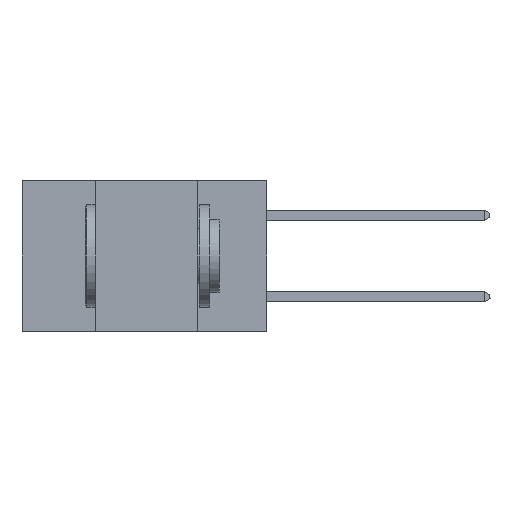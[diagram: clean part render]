
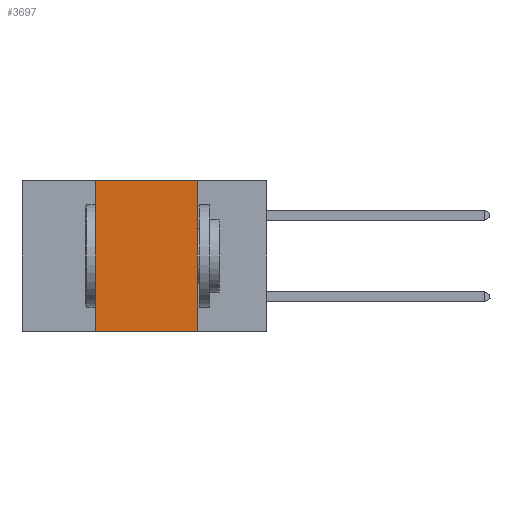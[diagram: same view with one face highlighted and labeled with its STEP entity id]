
A CAD part, left-side view. The second image highlights one B-rep face of the part: STEP entity #3697.
In plain terms, the highlighted planar face has unit normal (-1, 0, 0).
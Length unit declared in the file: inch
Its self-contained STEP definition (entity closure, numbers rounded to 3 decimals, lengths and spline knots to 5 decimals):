
#259 = DIRECTION ( 'NONE',  ( 1., 0., 0. ) ) ;
#348 = PLANE ( 'NONE',  #26039 ) ;
#994 = DIRECTION ( 'NONE',  ( 0., -1., 0. ) ) ;
#1923 = VERTEX_POINT ( 'NONE', #11440 ) ;
#2214 = ORIENTED_EDGE ( 'NONE', *, *, #6270, .T. ) ;
#3105 = DIRECTION ( 'NONE',  ( 0., 0., 1. ) ) ;
#3697 = ADVANCED_FACE ( 'NONE', ( #11895 ), #348, .F. ) ;
#4535 = DIRECTION ( 'NONE',  ( 0., 0., -1. ) ) ;
#4853 = VECTOR ( 'NONE', #19238, 39.37008 ) ;
#4961 = VECTOR ( 'NONE', #12912, 39.37008 ) ;
#5135 = CARTESIAN_POINT ( 'NONE',  ( 0., 0.42, 0. ) ) ;
#5522 = VERTEX_POINT ( 'NONE', #5718 ) ;
#5718 = CARTESIAN_POINT ( 'NONE',  ( 0., 0.17, 0. ) ) ;
#6270 = EDGE_CURVE ( 'NONE', #17530, #27174, #6605, .T. ) ;
#6420 = VECTOR ( 'NONE', #3105, 39.37008 ) ;
#6551 = EDGE_CURVE ( 'NONE', #5522, #27174, #23052, .T. ) ;
#6605 = LINE ( 'NONE', #9793, #17155 ) ;
#6617 = CARTESIAN_POINT ( 'NONE',  ( 0., 0.17, -0.37 ) ) ;
#8066 = CARTESIAN_POINT ( 'NONE',  ( 0., 0.42, -0.37 ) ) ;
#9050 = CARTESIAN_POINT ( 'NONE',  ( 0., 0.17, 0. ) ) ;
#9793 = CARTESIAN_POINT ( 'NONE',  ( 0., 0.6, -0.37 ) ) ;
#11440 = CARTESIAN_POINT ( 'NONE',  ( 0., 0.42, 0. ) ) ;
#11895 = FACE_OUTER_BOUND ( 'NONE', #13043, .T. ) ;
#12380 = ORIENTED_EDGE ( 'NONE', *, *, #6551, .F. ) ;
#12830 = CARTESIAN_POINT ( 'NONE',  ( 0., 0.6, 0. ) ) ;
#12912 = DIRECTION ( 'NONE',  ( 0., 0., -1. ) ) ;
#13043 = EDGE_LOOP ( 'NONE', ( #12380, #19731, #19975, #2214 ) ) ;
#16315 = LINE ( 'NONE', #5135, #6420 ) ;
#17155 = VECTOR ( 'NONE', #994, 39.37008 ) ;
#17242 = CARTESIAN_POINT ( 'NONE',  ( 0., 0.6, 0. ) ) ;
#17530 = VERTEX_POINT ( 'NONE', #8066 ) ;
#18865 = EDGE_CURVE ( 'NONE', #1923, #5522, #25599, .T. ) ;
#19238 = DIRECTION ( 'NONE',  ( 0., -1., 0. ) ) ;
#19731 = ORIENTED_EDGE ( 'NONE', *, *, #18865, .F. ) ;
#19975 = ORIENTED_EDGE ( 'NONE', *, *, #20944, .F. ) ;
#20944 = EDGE_CURVE ( 'NONE', #17530, #1923, #16315, .T. ) ;
#23052 = LINE ( 'NONE', #9050, #4961 ) ;
#25599 = LINE ( 'NONE', #17242, #4853 ) ;
#26039 = AXIS2_PLACEMENT_3D ( 'NONE', #12830, #259, #4535 ) ;
#27174 = VERTEX_POINT ( 'NONE', #6617 ) ;
